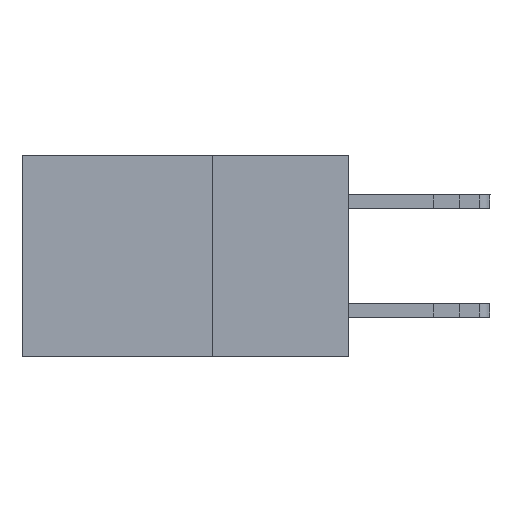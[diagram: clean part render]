
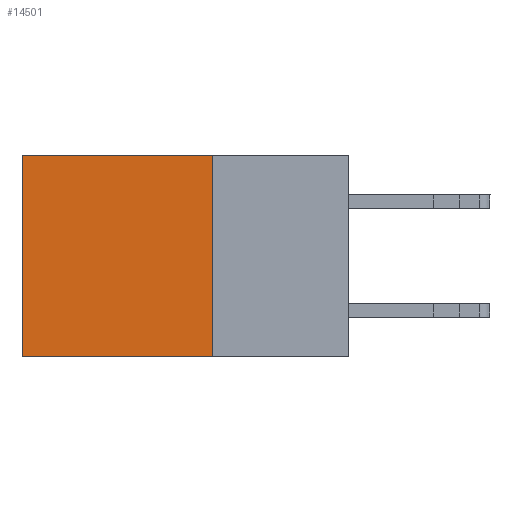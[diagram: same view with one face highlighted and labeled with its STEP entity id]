
A CAD part, left-side view. The second image highlights one B-rep face of the part: STEP entity #14501.
In plain terms, the highlighted planar face has unit normal (-1, 0, 0).
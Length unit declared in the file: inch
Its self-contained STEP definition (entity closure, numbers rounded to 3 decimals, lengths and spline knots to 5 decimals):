
#61 = ORIENTED_EDGE ( 'NONE', *, *, #4708, .T. ) ;
#205 = LINE ( 'NONE', #448, #10845 ) ;
#448 = CARTESIAN_POINT ( 'NONE',  ( 0.298, 0.25, -0.37 ) ) ;
#474 = LINE ( 'NONE', #1215, #15185 ) ;
#1215 = CARTESIAN_POINT ( 'NONE',  ( 0.298, 0.25, 0. ) ) ;
#1935 = ORIENTED_EDGE ( 'NONE', *, *, #2219, .T. ) ;
#2196 = CARTESIAN_POINT ( 'NONE',  ( 0.298, 0.25, -0.37 ) ) ;
#2219 = EDGE_CURVE ( 'NONE', #13655, #6451, #474, .T. ) ;
#2519 = CARTESIAN_POINT ( 'NONE',  ( 0.298, 0.6, 0. ) ) ;
#2575 = DIRECTION ( 'NONE',  ( 1., 0., 0. ) ) ;
#2619 = DIRECTION ( 'NONE',  ( 0., 0., -1. ) ) ;
#2754 = DIRECTION ( 'NONE',  ( 0., 1., 0. ) ) ;
#3055 = DIRECTION ( 'NONE',  ( 0., 0., -1. ) ) ;
#3542 = DIRECTION ( 'NONE',  ( 0., 1., 0. ) ) ;
#4292 = EDGE_CURVE ( 'NONE', #13655, #5623, #8153, .T. ) ;
#4490 = ORIENTED_EDGE ( 'NONE', *, *, #11857, .F. ) ;
#4708 = EDGE_CURVE ( 'NONE', #6451, #11212, #10790, .T. ) ;
#5294 = CARTESIAN_POINT ( 'NONE',  ( 0.298, 0.25, 0. ) ) ;
#5623 = VERTEX_POINT ( 'NONE', #2196 ) ;
#6294 = FACE_OUTER_BOUND ( 'NONE', #13420, .T. ) ;
#6451 = VERTEX_POINT ( 'NONE', #17086 ) ;
#6856 = CARTESIAN_POINT ( 'NONE',  ( 0.298, 0.6, -0.37 ) ) ;
#8153 = LINE ( 'NONE', #5294, #15104 ) ;
#9416 = VECTOR ( 'NONE', #2619, 39.37008 ) ;
#10790 = LINE ( 'NONE', #2519, #9416 ) ;
#10845 = VECTOR ( 'NONE', #3542, 39.37008 ) ;
#11107 = CARTESIAN_POINT ( 'NONE',  ( 0.298, 0.25, 0. ) ) ;
#11212 = VERTEX_POINT ( 'NONE', #6856 ) ;
#11857 = EDGE_CURVE ( 'NONE', #5623, #11212, #205, .T. ) ;
#12463 = DIRECTION ( 'NONE',  ( 0., 0., -1. ) ) ;
#13059 = CARTESIAN_POINT ( 'NONE',  ( 0.298, 0.25, 0. ) ) ;
#13237 = ORIENTED_EDGE ( 'NONE', *, *, #4292, .F. ) ;
#13420 = EDGE_LOOP ( 'NONE', ( #61, #4490, #13237, #1935 ) ) ;
#13655 = VERTEX_POINT ( 'NONE', #13059 ) ;
#14501 = ADVANCED_FACE ( 'NONE', ( #6294 ), #16602, .F. ) ;
#15104 = VECTOR ( 'NONE', #3055, 39.37008 ) ;
#15185 = VECTOR ( 'NONE', #2754, 39.37008 ) ;
#16602 = PLANE ( 'NONE',  #18245 ) ;
#17086 = CARTESIAN_POINT ( 'NONE',  ( 0.298, 0.6, 0. ) ) ;
#18245 = AXIS2_PLACEMENT_3D ( 'NONE', #11107, #2575, #12463 ) ;
